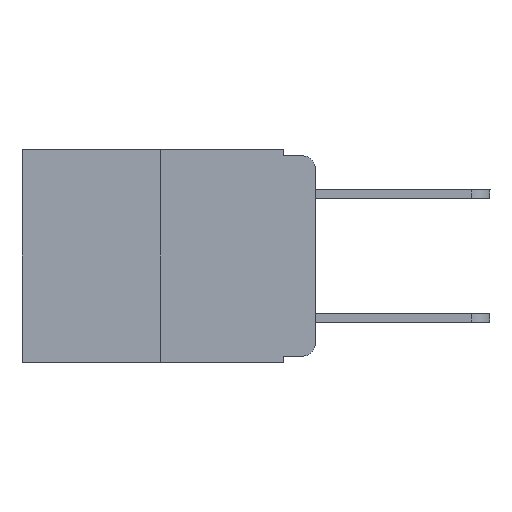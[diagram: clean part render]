
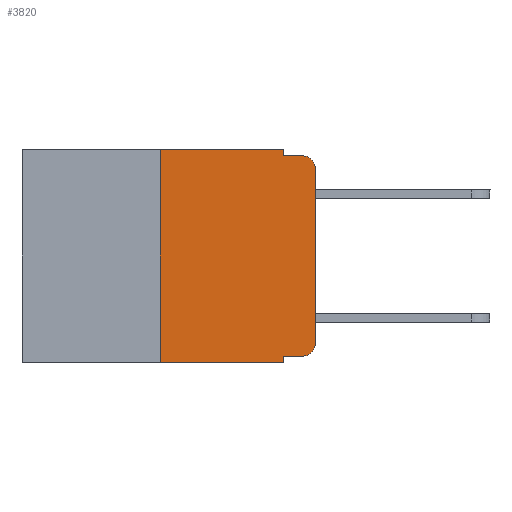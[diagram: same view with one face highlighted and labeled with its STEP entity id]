
A CAD part, left-side view. The second image highlights one B-rep face of the part: STEP entity #3820.
In plain terms, the highlighted planar face has unit normal (-1, 0, 0).
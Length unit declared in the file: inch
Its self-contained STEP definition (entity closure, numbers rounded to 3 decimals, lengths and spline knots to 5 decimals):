
#26 = VERTEX_POINT ( 'NONE', #10352 ) ;
#126 = ORIENTED_EDGE ( 'NONE', *, *, #1059, .T. ) ;
#580 = CARTESIAN_POINT ( 'NONE',  ( 0., 0.051, 0. ) ) ;
#590 = DIRECTION ( 'NONE',  ( 0., 0., -1. ) ) ;
#766 = LINE ( 'NONE', #15336, #16646 ) ;
#809 = AXIS2_PLACEMENT_3D ( 'NONE', #12530, #2722, #590 ) ;
#1059 = EDGE_CURVE ( 'NONE', #15774, #12871, #19677, .T. ) ;
#1343 = ORIENTED_EDGE ( 'NONE', *, *, #25868, .F. ) ;
#1517 = CARTESIAN_POINT ( 'NONE',  ( 0., 0.051, -0.333 ) ) ;
#2142 = DIRECTION ( 'NONE',  ( 0., -1., 0. ) ) ;
#2209 = VERTEX_POINT ( 'NONE', #10564 ) ;
#2384 = VERTEX_POINT ( 'NONE', #9080 ) ;
#2722 = DIRECTION ( 'NONE',  ( 1., 0., 0. ) ) ;
#3139 = DIRECTION ( 'NONE',  ( 0., 0., 1. ) ) ;
#3306 = ORIENTED_EDGE ( 'NONE', *, *, #21408, .F. ) ;
#3617 = CARTESIAN_POINT ( 'NONE',  ( 0., 0., -0.03 ) ) ;
#3820 = ADVANCED_FACE ( 'NONE', ( #23023 ), #10663, .F. ) ;
#4040 = VECTOR ( 'NONE', #8670, 39.37008 ) ;
#4772 = VERTEX_POINT ( 'NONE', #5309 ) ;
#4844 = EDGE_CURVE ( 'NONE', #12871, #2209, #19315, .T. ) ;
#5136 = LINE ( 'NONE', #13329, #22488 ) ;
#5225 = CARTESIAN_POINT ( 'NONE',  ( 0., 0.051, -0.01 ) ) ;
#5309 = CARTESIAN_POINT ( 'NONE',  ( 0., 0.051, 0. ) ) ;
#5509 = CARTESIAN_POINT ( 'NONE',  ( 0., 0.02, -0.03 ) ) ;
#5837 = DIRECTION ( 'NONE',  ( 0., -1., 0. ) ) ;
#6012 = CARTESIAN_POINT ( 'NONE',  ( 0., 0.051, -0.01 ) ) ;
#6524 = EDGE_CURVE ( 'NONE', #11255, #2384, #766, .T. ) ;
#7456 = VERTEX_POINT ( 'NONE', #5225 ) ;
#7493 = DIRECTION ( 'NONE',  ( 0., 0., -1. ) ) ;
#8181 = VECTOR ( 'NONE', #5837, 39.37008 ) ;
#8449 = CARTESIAN_POINT ( 'NONE',  ( 0., 0.051, 0. ) ) ;
#8670 = DIRECTION ( 'NONE',  ( 0., 0., -1. ) ) ;
#8688 = EDGE_CURVE ( 'NONE', #11255, #23291, #5136, .T. ) ;
#9080 = CARTESIAN_POINT ( 'NONE',  ( 0., 0.051, -0.343 ) ) ;
#9975 = LINE ( 'NONE', #6012, #19051 ) ;
#10299 = ORIENTED_EDGE ( 'NONE', *, *, #20402, .F. ) ;
#10352 = CARTESIAN_POINT ( 'NONE',  ( 0., 0.02, -0.01 ) ) ;
#10564 = CARTESIAN_POINT ( 'NONE',  ( 0., 0., -0.313 ) ) ;
#10646 = DIRECTION ( 'NONE',  ( 0., 0., 1. ) ) ;
#10663 = PLANE ( 'NONE',  #809 ) ;
#11039 = CARTESIAN_POINT ( 'NONE',  ( 0., 0., 0. ) ) ;
#11159 = LINE ( 'NONE', #11039, #21495 ) ;
#11255 = VERTEX_POINT ( 'NONE', #26224 ) ;
#11429 = CARTESIAN_POINT ( 'NONE',  ( 0., 0.051, -0.333 ) ) ;
#11779 = EDGE_CURVE ( 'NONE', #23291, #4772, #18176, .T. ) ;
#11852 = DIRECTION ( 'NONE',  ( -1., 0., 0. ) ) ;
#11854 = ORIENTED_EDGE ( 'NONE', *, *, #6524, .T. ) ;
#11890 = ORIENTED_EDGE ( 'NONE', *, *, #17384, .T. ) ;
#12530 = CARTESIAN_POINT ( 'NONE',  ( 0., 0.473, 0. ) ) ;
#12553 = LINE ( 'NONE', #8449, #23700 ) ;
#12830 = EDGE_LOOP ( 'NONE', ( #11890, #24313, #3306, #1343, #14837, #18524, #11854, #10299, #126, #19364 ) ) ;
#12871 = VERTEX_POINT ( 'NONE', #22903 ) ;
#13329 = CARTESIAN_POINT ( 'NONE',  ( 0., 0.25, 0. ) ) ;
#13382 = AXIS2_PLACEMENT_3D ( 'NONE', #19089, #23226, #23095 ) ;
#13504 = CARTESIAN_POINT ( 'NONE',  ( 0., 0.25, 0. ) ) ;
#14480 = DIRECTION ( 'NONE',  ( 0., -1., 0. ) ) ;
#14837 = ORIENTED_EDGE ( 'NONE', *, *, #11779, .F. ) ;
#15209 = DIRECTION ( 'NONE',  ( 0., -1., 0. ) ) ;
#15336 = CARTESIAN_POINT ( 'NONE',  ( 0., 0.473, -0.343 ) ) ;
#15774 = VERTEX_POINT ( 'NONE', #11429 ) ;
#16646 = VECTOR ( 'NONE', #15209, 39.37008 ) ;
#17384 = EDGE_CURVE ( 'NONE', #2209, #24757, #11159, .T. ) ;
#18176 = LINE ( 'NONE', #20564, #8181 ) ;
#18494 = EDGE_CURVE ( 'NONE', #24757, #26, #22328, .T. ) ;
#18524 = ORIENTED_EDGE ( 'NONE', *, *, #8688, .F. ) ;
#18756 = LINE ( 'NONE', #580, #4040 ) ;
#19051 = VECTOR ( 'NONE', #14480, 39.37008 ) ;
#19089 = CARTESIAN_POINT ( 'NONE',  ( 0., 0.02, -0.313 ) ) ;
#19315 = CIRCLE ( 'NONE', #13382, 0.02 ) ;
#19364 = ORIENTED_EDGE ( 'NONE', *, *, #4844, .T. ) ;
#19677 = LINE ( 'NONE', #1517, #21010 ) ;
#20402 = EDGE_CURVE ( 'NONE', #15774, #2384, #12553, .T. ) ;
#20564 = CARTESIAN_POINT ( 'NONE',  ( 0., 0.473, 0. ) ) ;
#21010 = VECTOR ( 'NONE', #2142, 39.37008 ) ;
#21408 = EDGE_CURVE ( 'NONE', #7456, #26, #9975, .T. ) ;
#21495 = VECTOR ( 'NONE', #10646, 39.37008 ) ;
#22328 = CIRCLE ( 'NONE', #25730, 0.02 ) ;
#22488 = VECTOR ( 'NONE', #3139, 39.37008 ) ;
#22903 = CARTESIAN_POINT ( 'NONE',  ( 0., 0.02, -0.333 ) ) ;
#22919 = DIRECTION ( 'NONE',  ( 0., 0., -1. ) ) ;
#23023 = FACE_OUTER_BOUND ( 'NONE', #12830, .T. ) ;
#23095 = DIRECTION ( 'NONE',  ( 0., 0., -1. ) ) ;
#23226 = DIRECTION ( 'NONE',  ( -1., 0., 0. ) ) ;
#23291 = VERTEX_POINT ( 'NONE', #13504 ) ;
#23700 = VECTOR ( 'NONE', #22919, 39.37008 ) ;
#24313 = ORIENTED_EDGE ( 'NONE', *, *, #18494, .T. ) ;
#24757 = VERTEX_POINT ( 'NONE', #3617 ) ;
#25730 = AXIS2_PLACEMENT_3D ( 'NONE', #5509, #11852, #7493 ) ;
#25868 = EDGE_CURVE ( 'NONE', #4772, #7456, #18756, .T. ) ;
#26224 = CARTESIAN_POINT ( 'NONE',  ( 0., 0.25, -0.343 ) ) ;
